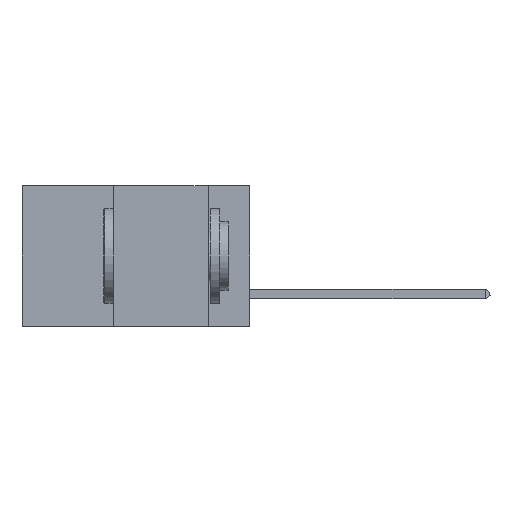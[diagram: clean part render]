
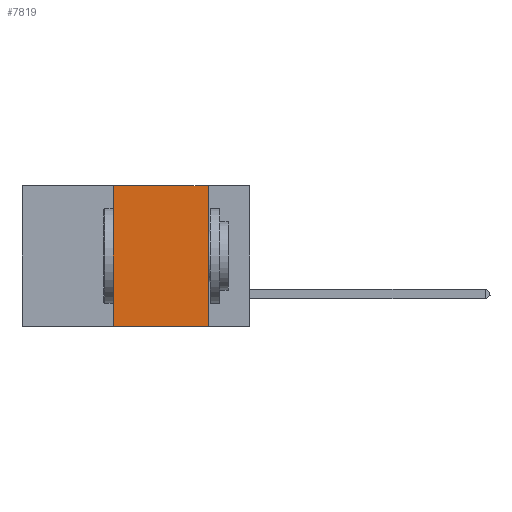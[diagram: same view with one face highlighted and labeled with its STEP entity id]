
A CAD part, left-side view. The second image highlights one B-rep face of the part: STEP entity #7819.
In plain terms, the highlighted planar face has unit normal (-1, 0, 0).
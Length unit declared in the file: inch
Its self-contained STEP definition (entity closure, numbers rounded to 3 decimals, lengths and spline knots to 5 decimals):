
#435 = LINE ( 'NONE', #5698, #10976 ) ;
#673 = LINE ( 'NONE', #9043, #3057 ) ;
#900 = EDGE_LOOP ( 'NONE', ( #7405, #1002, #8907, #2216 ) ) ;
#1002 = ORIENTED_EDGE ( 'NONE', *, *, #11755, .F. ) ;
#1165 = EDGE_CURVE ( 'NONE', #2644, #12667, #435, .T. ) ;
#1444 = CARTESIAN_POINT ( 'NONE',  ( 0., 0.6, 0. ) ) ;
#1531 = DIRECTION ( 'NONE',  ( 0., 0., -1. ) ) ;
#2095 = VERTEX_POINT ( 'NONE', #8451 ) ;
#2216 = ORIENTED_EDGE ( 'NONE', *, *, #10452, .T. ) ;
#2644 = VERTEX_POINT ( 'NONE', #13229 ) ;
#3057 = VECTOR ( 'NONE', #3192, 39.37008 ) ;
#3192 = DIRECTION ( 'NONE',  ( 0., 0., 1. ) ) ;
#3683 = EDGE_CURVE ( 'NONE', #13004, #2095, #673, .T. ) ;
#4311 = AXIS2_PLACEMENT_3D ( 'NONE', #1444, #9604, #1531 ) ;
#4621 = FACE_OUTER_BOUND ( 'NONE', #900, .T. ) ;
#4660 = PLANE ( 'NONE',  #4311 ) ;
#5195 = CARTESIAN_POINT ( 'NONE',  ( 0., 0.6, -0.37 ) ) ;
#5448 = DIRECTION ( 'NONE',  ( 0., -1., 0. ) ) ;
#5698 = CARTESIAN_POINT ( 'NONE',  ( 0., 0.11, 0. ) ) ;
#7097 = CARTESIAN_POINT ( 'NONE',  ( 0., 0.36, -0.37 ) ) ;
#7405 = ORIENTED_EDGE ( 'NONE', *, *, #1165, .F. ) ;
#7819 = ADVANCED_FACE ( 'NONE', ( #4621 ), #4660, .F. ) ;
#7914 = VECTOR ( 'NONE', #12333, 39.37008 ) ;
#8451 = CARTESIAN_POINT ( 'NONE',  ( 0., 0.36, 0. ) ) ;
#8494 = CARTESIAN_POINT ( 'NONE',  ( 0., 0.6, 0. ) ) ;
#8907 = ORIENTED_EDGE ( 'NONE', *, *, #3683, .F. ) ;
#8982 = LINE ( 'NONE', #8494, #9778 ) ;
#9043 = CARTESIAN_POINT ( 'NONE',  ( 0., 0.36, 0. ) ) ;
#9604 = DIRECTION ( 'NONE',  ( 1., 0., 0. ) ) ;
#9778 = VECTOR ( 'NONE', #5448, 39.37008 ) ;
#10253 = CARTESIAN_POINT ( 'NONE',  ( 0., 0.11, -0.37 ) ) ;
#10452 = EDGE_CURVE ( 'NONE', #13004, #12667, #11893, .T. ) ;
#10941 = DIRECTION ( 'NONE',  ( 0., 0., -1. ) ) ;
#10976 = VECTOR ( 'NONE', #10941, 39.37008 ) ;
#11755 = EDGE_CURVE ( 'NONE', #2095, #2644, #8982, .T. ) ;
#11893 = LINE ( 'NONE', #5195, #7914 ) ;
#12333 = DIRECTION ( 'NONE',  ( 0., -1., 0. ) ) ;
#12667 = VERTEX_POINT ( 'NONE', #10253 ) ;
#13004 = VERTEX_POINT ( 'NONE', #7097 ) ;
#13229 = CARTESIAN_POINT ( 'NONE',  ( 0., 0.11, 0. ) ) ;
